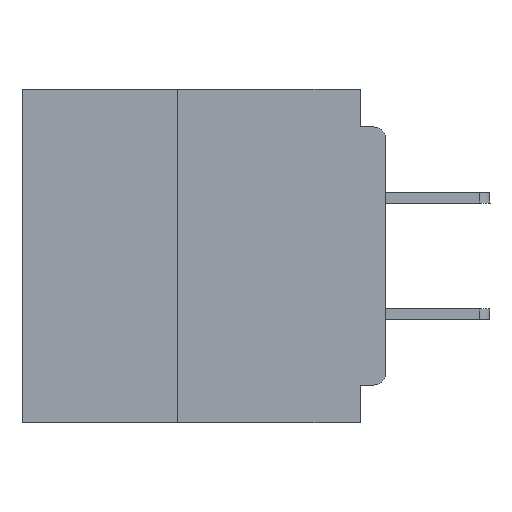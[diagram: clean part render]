
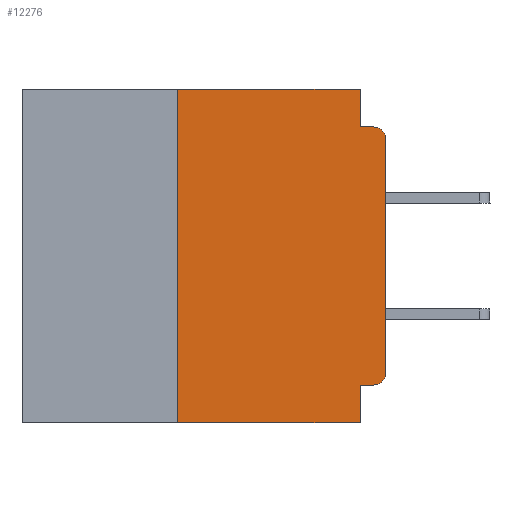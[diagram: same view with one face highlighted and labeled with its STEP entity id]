
A CAD part, left-side view. The second image highlights one B-rep face of the part: STEP entity #12276.
In plain terms, the highlighted planar face has unit normal (-1, 0, 0).
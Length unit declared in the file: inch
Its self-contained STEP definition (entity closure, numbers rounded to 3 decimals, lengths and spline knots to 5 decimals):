
#253 = CARTESIAN_POINT ( 'NONE',  ( 0., 0., -0.355 ) ) ;
#2421 = CIRCLE ( 'NONE', #42642, 0.015 ) ;
#2467 = EDGE_CURVE ( 'NONE', #60891, #43038, #31446, .T. ) ;
#2731 = CARTESIAN_POINT ( 'NONE',  ( 0., 0., 0. ) ) ;
#3323 = CARTESIAN_POINT ( 'NONE',  ( 0., 0.031, 0. ) ) ;
#3659 = DIRECTION ( 'NONE',  ( 0., 0., -1. ) ) ;
#3876 = LINE ( 'NONE', #55793, #40841 ) ;
#5182 = CARTESIAN_POINT ( 'NONE',  ( 0., 0.015, -0.355 ) ) ;
#5260 = CARTESIAN_POINT ( 'NONE',  ( 0., 0.031, -0.4 ) ) ;
#5320 = ORIENTED_EDGE ( 'NONE', *, *, #63313, .F. ) ;
#5706 = CARTESIAN_POINT ( 'NONE',  ( 0., 0.031, -0.045 ) ) ;
#5796 = VECTOR ( 'NONE', #63240, 39.37008 ) ;
#7713 = CARTESIAN_POINT ( 'NONE',  ( 0., 0., -0.34 ) ) ;
#7858 = EDGE_CURVE ( 'NONE', #63830, #14732, #63352, .T. ) ;
#9162 = EDGE_CURVE ( 'NONE', #43038, #48160, #27442, .T. ) ;
#10317 = AXIS2_PLACEMENT_3D ( 'NONE', #44454, #49436, #19437 ) ;
#10431 = DIRECTION ( 'NONE',  ( 0., 1., 0. ) ) ;
#11561 = CARTESIAN_POINT ( 'NONE',  ( 0., 0., -0.045 ) ) ;
#12276 = ADVANCED_FACE ( 'NONE', ( #29228 ), #34425, .F. ) ;
#12888 = DIRECTION ( 'NONE',  ( 0., 0., 1. ) ) ;
#13713 = DIRECTION ( 'NONE',  ( -1., 0., 0. ) ) ;
#14732 = VERTEX_POINT ( 'NONE', #17798 ) ;
#16080 = AXIS2_PLACEMENT_3D ( 'NONE', #43787, #13713, #48758 ) ;
#17039 = EDGE_CURVE ( 'NONE', #28986, #52641, #23047, .T. ) ;
#17798 = CARTESIAN_POINT ( 'NONE',  ( 0., 0.031, -0.355 ) ) ;
#18080 = VECTOR ( 'NONE', #12888, 39.37008 ) ;
#18469 = ORIENTED_EDGE ( 'NONE', *, *, #44164, .F. ) ;
#19437 = DIRECTION ( 'NONE',  ( 0., 0., -1. ) ) ;
#23047 = LINE ( 'NONE', #25209, #34876 ) ;
#23221 = CARTESIAN_POINT ( 'NONE',  ( 0., 0., -0.06 ) ) ;
#23593 = EDGE_CURVE ( 'NONE', #28986, #35772, #61014, .T. ) ;
#24046 = ORIENTED_EDGE ( 'NONE', *, *, #47428, .T. ) ;
#24794 = CARTESIAN_POINT ( 'NONE',  ( 0., 0.25, -0.4 ) ) ;
#25209 = CARTESIAN_POINT ( 'NONE',  ( 0., 0.437, -0.4 ) ) ;
#25237 = ORIENTED_EDGE ( 'NONE', *, *, #23593, .F. ) ;
#25695 = VECTOR ( 'NONE', #45473, 39.37008 ) ;
#27442 = CIRCLE ( 'NONE', #16080, 0.015 ) ;
#28986 = VERTEX_POINT ( 'NONE', #24794 ) ;
#29228 = FACE_OUTER_BOUND ( 'NONE', #47660, .T. ) ;
#29732 = EDGE_CURVE ( 'NONE', #51043, #48160, #34501, .T. ) ;
#30286 = DIRECTION ( 'NONE',  ( 0., -1., 0. ) ) ;
#31401 = CARTESIAN_POINT ( 'NONE',  ( 0., 0.25, -0.4 ) ) ;
#31446 = LINE ( 'NONE', #2731, #18080 ) ;
#32593 = LINE ( 'NONE', #3323, #5796 ) ;
#33831 = DIRECTION ( 'NONE',  ( -1., 0., 0. ) ) ;
#34425 = PLANE ( 'NONE',  #10317 ) ;
#34501 = LINE ( 'NONE', #11561, #46214 ) ;
#34876 = VECTOR ( 'NONE', #30286, 39.37008 ) ;
#35772 = VERTEX_POINT ( 'NONE', #36349 ) ;
#36111 = DIRECTION ( 'NONE',  ( 0., -1., 0. ) ) ;
#36349 = CARTESIAN_POINT ( 'NONE',  ( 0., 0.25, 0. ) ) ;
#39092 = LINE ( 'NONE', #5260, #25695 ) ;
#40841 = VECTOR ( 'NONE', #36111, 39.37008 ) ;
#41497 = DIRECTION ( 'NONE',  ( 0., 0., 1. ) ) ;
#41637 = DIRECTION ( 'NONE',  ( 0., -1., 0. ) ) ;
#42642 = AXIS2_PLACEMENT_3D ( 'NONE', #63556, #33831, #3659 ) ;
#43038 = VERTEX_POINT ( 'NONE', #23221 ) ;
#43363 = ORIENTED_EDGE ( 'NONE', *, *, #29732, .F. ) ;
#43787 = CARTESIAN_POINT ( 'NONE',  ( 0., 0.015, -0.06 ) ) ;
#44164 = EDGE_CURVE ( 'NONE', #14732, #52641, #39092, .T. ) ;
#44454 = CARTESIAN_POINT ( 'NONE',  ( 0., 0.437, 0. ) ) ;
#45473 = DIRECTION ( 'NONE',  ( 0., 0., -1. ) ) ;
#46214 = VECTOR ( 'NONE', #41637, 39.37008 ) ;
#47428 = EDGE_CURVE ( 'NONE', #63830, #60891, #2421, .T. ) ;
#47660 = EDGE_LOOP ( 'NONE', ( #58138, #63697, #43363, #51485, #5320, #25237, #50110, #18469, #60289, #24046 ) ) ;
#48160 = VERTEX_POINT ( 'NONE', #59574 ) ;
#48758 = DIRECTION ( 'NONE',  ( 0., 0., -1. ) ) ;
#48943 = EDGE_CURVE ( 'NONE', #52393, #51043, #32593, .T. ) ;
#49436 = DIRECTION ( 'NONE',  ( 1., 0., 0. ) ) ;
#50110 = ORIENTED_EDGE ( 'NONE', *, *, #17039, .T. ) ;
#50932 = VECTOR ( 'NONE', #41497, 39.37008 ) ;
#51043 = VERTEX_POINT ( 'NONE', #5706 ) ;
#51485 = ORIENTED_EDGE ( 'NONE', *, *, #48943, .F. ) ;
#52393 = VERTEX_POINT ( 'NONE', #61175 ) ;
#52641 = VERTEX_POINT ( 'NONE', #58287 ) ;
#53272 = VECTOR ( 'NONE', #10431, 39.37008 ) ;
#55793 = CARTESIAN_POINT ( 'NONE',  ( 0., 0.437, 0. ) ) ;
#58138 = ORIENTED_EDGE ( 'NONE', *, *, #2467, .T. ) ;
#58287 = CARTESIAN_POINT ( 'NONE',  ( 0., 0.031, -0.4 ) ) ;
#59574 = CARTESIAN_POINT ( 'NONE',  ( 0., 0.015, -0.045 ) ) ;
#60289 = ORIENTED_EDGE ( 'NONE', *, *, #7858, .F. ) ;
#60891 = VERTEX_POINT ( 'NONE', #7713 ) ;
#61014 = LINE ( 'NONE', #31401, #50932 ) ;
#61175 = CARTESIAN_POINT ( 'NONE',  ( 0., 0.031, 0. ) ) ;
#63240 = DIRECTION ( 'NONE',  ( 0., 0., -1. ) ) ;
#63313 = EDGE_CURVE ( 'NONE', #35772, #52393, #3876, .T. ) ;
#63352 = LINE ( 'NONE', #253, #53272 ) ;
#63556 = CARTESIAN_POINT ( 'NONE',  ( 0., 0.015, -0.34 ) ) ;
#63697 = ORIENTED_EDGE ( 'NONE', *, *, #9162, .T. ) ;
#63830 = VERTEX_POINT ( 'NONE', #5182 ) ;
